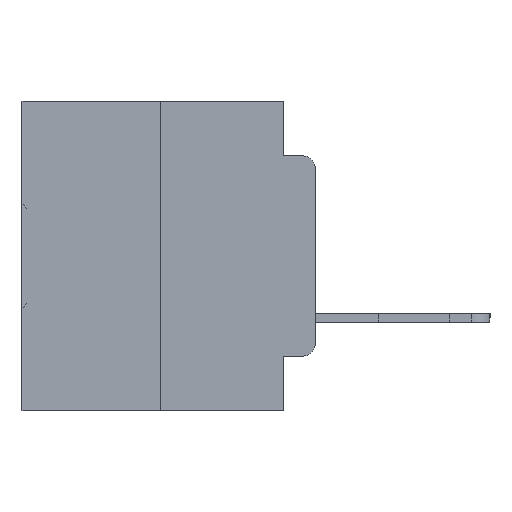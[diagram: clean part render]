
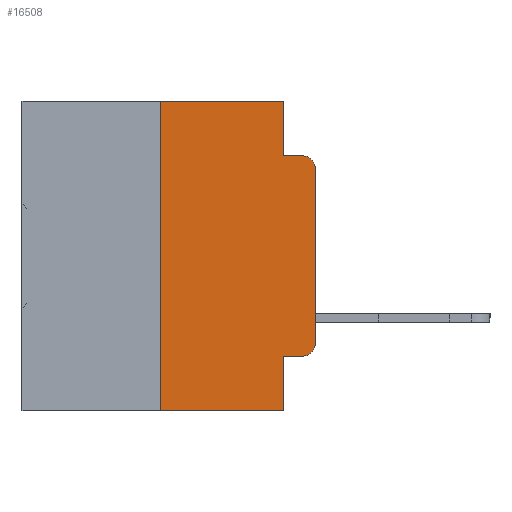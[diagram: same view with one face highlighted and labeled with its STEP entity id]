
A CAD part, left-side view. The second image highlights one B-rep face of the part: STEP entity #16508.
In plain terms, the highlighted planar face has unit normal (-1, 0, 0).
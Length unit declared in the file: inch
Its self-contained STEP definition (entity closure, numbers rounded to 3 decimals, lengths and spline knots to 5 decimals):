
#159 = CARTESIAN_POINT ( 'NONE',  ( 0., 0.051, -0.4115 ) ) ;
#248 = ORIENTED_EDGE ( 'NONE', *, *, #11705, .T. ) ;
#497 = VERTEX_POINT ( 'NONE', #21263 ) ;
#903 = EDGE_CURVE ( 'NONE', #22012, #24354, #27319, .T. ) ;
#907 = VECTOR ( 'NONE', #22409, 39.37008 ) ;
#1105 = VERTEX_POINT ( 'NONE', #21350 ) ;
#1842 = DIRECTION ( 'NONE',  ( 0., 0., -1. ) ) ;
#2874 = ORIENTED_EDGE ( 'NONE', *, *, #30137, .F. ) ;
#2910 = PLANE ( 'NONE',  #24718 ) ;
#3232 = LINE ( 'NONE', #159, #28669 ) ;
#3246 = AXIS2_PLACEMENT_3D ( 'NONE', #13443, #30711, #15986 ) ;
#3873 = LINE ( 'NONE', #25923, #14654 ) ;
#3921 = ORIENTED_EDGE ( 'NONE', *, *, #27415, .T. ) ;
#4072 = VECTOR ( 'NONE', #27530, 39.37008 ) ;
#4270 = EDGE_CURVE ( 'NONE', #28433, #30860, #3873, .T. ) ;
#5407 = CARTESIAN_POINT ( 'NONE',  ( 0., 0.473, 0. ) ) ;
#5492 = VERTEX_POINT ( 'NONE', #20020 ) ;
#5753 = VECTOR ( 'NONE', #22273, 39.37008 ) ;
#5874 = VERTEX_POINT ( 'NONE', #17972 ) ;
#6113 = ORIENTED_EDGE ( 'NONE', *, *, #20825, .F. ) ;
#6323 = CARTESIAN_POINT ( 'NONE',  ( 0., 0., -0.1085 ) ) ;
#7246 = VERTEX_POINT ( 'NONE', #13758 ) ;
#7910 = DIRECTION ( 'NONE',  ( 1., 0., 0. ) ) ;
#7991 = EDGE_LOOP ( 'NONE', ( #3921, #8486, #6113, #8726, #2874, #24803, #248, #15267, #26897, #15382 ) ) ;
#8486 = ORIENTED_EDGE ( 'NONE', *, *, #25763, .T. ) ;
#8726 = ORIENTED_EDGE ( 'NONE', *, *, #12485, .F. ) ;
#8960 = DIRECTION ( 'NONE',  ( 0., -1., 0. ) ) ;
#10255 = VECTOR ( 'NONE', #8960, 39.37008 ) ;
#10660 = AXIS2_PLACEMENT_3D ( 'NONE', #31440, #16707, #1842 ) ;
#11705 = EDGE_CURVE ( 'NONE', #28433, #24354, #25434, .T. ) ;
#12485 = EDGE_CURVE ( 'NONE', #5492, #497, #28445, .T. ) ;
#13098 = CIRCLE ( 'NONE', #10660, 0.02 ) ;
#13443 = CARTESIAN_POINT ( 'NONE',  ( 0., 0.02, -0.1085 ) ) ;
#13758 = CARTESIAN_POINT ( 'NONE',  ( 0., 0.02, -0.4115 ) ) ;
#14654 = VECTOR ( 'NONE', #16757, 39.37008 ) ;
#14995 = CIRCLE ( 'NONE', #3246, 0.02 ) ;
#15267 = ORIENTED_EDGE ( 'NONE', *, *, #903, .F. ) ;
#15382 = ORIENTED_EDGE ( 'NONE', *, *, #24716, .T. ) ;
#15951 = CARTESIAN_POINT ( 'NONE',  ( 0., 0.051, -0.4115 ) ) ;
#15986 = DIRECTION ( 'NONE',  ( 0., 0., -1. ) ) ;
#16508 = ADVANCED_FACE ( 'NONE', ( #26291 ), #2910, .F. ) ;
#16707 = DIRECTION ( 'NONE',  ( -1., 0., 0. ) ) ;
#16757 = DIRECTION ( 'NONE',  ( 0., 0., 1. ) ) ;
#17548 = DIRECTION ( 'NONE',  ( 0., -1., 0. ) ) ;
#17972 = CARTESIAN_POINT ( 'NONE',  ( 0., 0., -0.3915 ) ) ;
#19800 = CARTESIAN_POINT ( 'NONE',  ( 0., 0.473, -0.5 ) ) ;
#20020 = CARTESIAN_POINT ( 'NONE',  ( 0., 0.051, 0. ) ) ;
#20463 = CARTESIAN_POINT ( 'NONE',  ( 0., 0.25, 0. ) ) ;
#20825 = EDGE_CURVE ( 'NONE', #497, #1105, #26426, .T. ) ;
#21134 = VECTOR ( 'NONE', #25892, 39.37008 ) ;
#21240 = CARTESIAN_POINT ( 'NONE',  ( 0., 0.473, 0. ) ) ;
#21263 = CARTESIAN_POINT ( 'NONE',  ( 0., 0.051, -0.0885 ) ) ;
#21350 = CARTESIAN_POINT ( 'NONE',  ( 0., 0.02, -0.0885 ) ) ;
#21930 = CARTESIAN_POINT ( 'NONE',  ( 0., 0.051, 0. ) ) ;
#21966 = DIRECTION ( 'NONE',  ( 0., 0., -1. ) ) ;
#22012 = VERTEX_POINT ( 'NONE', #15951 ) ;
#22105 = VERTEX_POINT ( 'NONE', #6323 ) ;
#22273 = DIRECTION ( 'NONE',  ( 0., -1., 0. ) ) ;
#22409 = DIRECTION ( 'NONE',  ( 0., -1., 0. ) ) ;
#23024 = CARTESIAN_POINT ( 'NONE',  ( 0., 0.051, -0.5 ) ) ;
#23419 = CARTESIAN_POINT ( 'NONE',  ( 0., 0.051, 0. ) ) ;
#23761 = LINE ( 'NONE', #25058, #4072 ) ;
#24354 = VERTEX_POINT ( 'NONE', #23024 ) ;
#24467 = CARTESIAN_POINT ( 'NONE',  ( 0., 0.25, -0.5 ) ) ;
#24716 = EDGE_CURVE ( 'NONE', #7246, #5874, #13098, .T. ) ;
#24718 = AXIS2_PLACEMENT_3D ( 'NONE', #5407, #7910, #25131 ) ;
#24803 = ORIENTED_EDGE ( 'NONE', *, *, #4270, .F. ) ;
#25058 = CARTESIAN_POINT ( 'NONE',  ( 0., 0., 0. ) ) ;
#25131 = DIRECTION ( 'NONE',  ( 0., 0., -1. ) ) ;
#25434 = LINE ( 'NONE', #19800, #5753 ) ;
#25763 = EDGE_CURVE ( 'NONE', #22105, #1105, #14995, .T. ) ;
#25892 = DIRECTION ( 'NONE',  ( 0., 0., -1. ) ) ;
#25923 = CARTESIAN_POINT ( 'NONE',  ( 0., 0.25, 0. ) ) ;
#26291 = FACE_OUTER_BOUND ( 'NONE', #7991, .T. ) ;
#26426 = LINE ( 'NONE', #27349, #907 ) ;
#26538 = VECTOR ( 'NONE', #21966, 39.37008 ) ;
#26897 = ORIENTED_EDGE ( 'NONE', *, *, #31330, .T. ) ;
#27319 = LINE ( 'NONE', #21930, #26538 ) ;
#27349 = CARTESIAN_POINT ( 'NONE',  ( 0., 0.051, -0.0885 ) ) ;
#27415 = EDGE_CURVE ( 'NONE', #5874, #22105, #23761, .T. ) ;
#27530 = DIRECTION ( 'NONE',  ( 0., 0., 1. ) ) ;
#28433 = VERTEX_POINT ( 'NONE', #24467 ) ;
#28445 = LINE ( 'NONE', #23419, #21134 ) ;
#28669 = VECTOR ( 'NONE', #17548, 39.37008 ) ;
#29905 = LINE ( 'NONE', #21240, #10255 ) ;
#30137 = EDGE_CURVE ( 'NONE', #30860, #5492, #29905, .T. ) ;
#30711 = DIRECTION ( 'NONE',  ( -1., 0., 0. ) ) ;
#30860 = VERTEX_POINT ( 'NONE', #20463 ) ;
#31330 = EDGE_CURVE ( 'NONE', #22012, #7246, #3232, .T. ) ;
#31440 = CARTESIAN_POINT ( 'NONE',  ( 0., 0.02, -0.3915 ) ) ;
